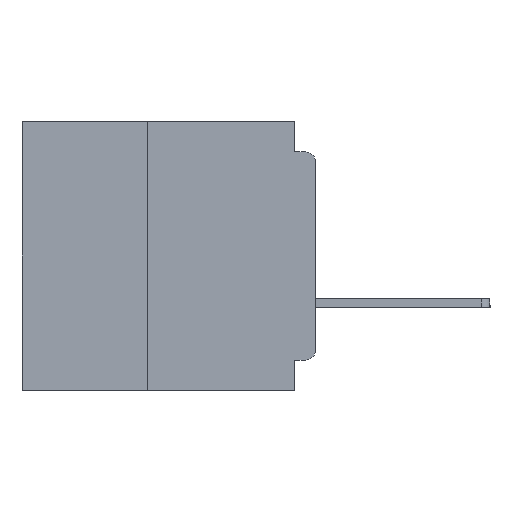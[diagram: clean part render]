
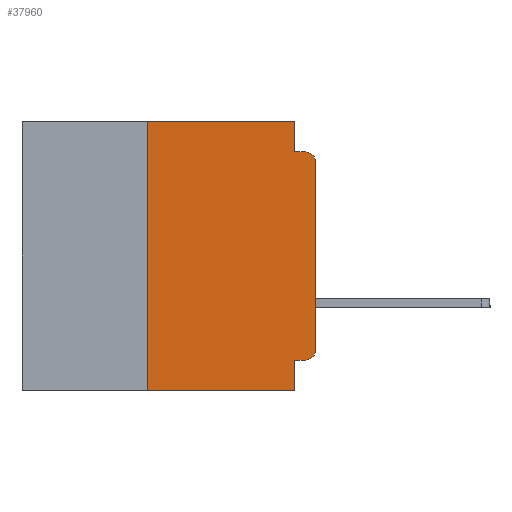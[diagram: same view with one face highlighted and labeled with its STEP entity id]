
A CAD part, left-side view. The second image highlights one B-rep face of the part: STEP entity #37960.
In plain terms, the highlighted planar face has unit normal (-1, 0, 0).
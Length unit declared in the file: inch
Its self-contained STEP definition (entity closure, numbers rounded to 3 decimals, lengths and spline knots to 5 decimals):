
#491 = ORIENTED_EDGE ( 'NONE', *, *, #46022, .F. ) ;
#1719 = VECTOR ( 'NONE', #11478, 39.37008 ) ;
#2384 = DIRECTION ( 'NONE',  ( 0., 1., 0. ) ) ;
#2435 = DIRECTION ( 'NONE',  ( 1., 0., 0. ) ) ;
#2574 = CARTESIAN_POINT ( 'NONE',  ( 0., 0., -0.355 ) ) ;
#2747 = VERTEX_POINT ( 'NONE', #2765 ) ;
#2765 = CARTESIAN_POINT ( 'NONE',  ( 0., 0., -0.34 ) ) ;
#3099 = DIRECTION ( 'NONE',  ( 0., -1., 0. ) ) ;
#3455 = CARTESIAN_POINT ( 'NONE',  ( 0., 0., -0.06 ) ) ;
#4271 = CIRCLE ( 'NONE', #40522, 0.015 ) ;
#4437 = EDGE_CURVE ( 'NONE', #35817, #33585, #36185, .T. ) ;
#5248 = VECTOR ( 'NONE', #12627, 39.37008 ) ;
#5250 = LINE ( 'NONE', #28716, #26916 ) ;
#6099 = VERTEX_POINT ( 'NONE', #3455 ) ;
#6126 = EDGE_CURVE ( 'NONE', #36416, #35817, #7019, .T. ) ;
#6572 = DIRECTION ( 'NONE',  ( 0., 0., 1. ) ) ;
#7019 = LINE ( 'NONE', #2574, #50005 ) ;
#8193 = EDGE_LOOP ( 'NONE', ( #16247, #42101, #491, #33173, #20647, #9060, #18084, #15968, #11695, #17584 ) ) ;
#9060 = ORIENTED_EDGE ( 'NONE', *, *, #16809, .F. ) ;
#10268 = PLANE ( 'NONE',  #50622 ) ;
#10523 = EDGE_CURVE ( 'NONE', #38878, #30469, #30773, .T. ) ;
#11369 = VERTEX_POINT ( 'NONE', #50577 ) ;
#11478 = DIRECTION ( 'NONE',  ( 0., 0., -1. ) ) ;
#11664 = CARTESIAN_POINT ( 'NONE',  ( 0., 0.031, -0.4 ) ) ;
#11695 = ORIENTED_EDGE ( 'NONE', *, *, #6126, .F. ) ;
#12627 = DIRECTION ( 'NONE',  ( 0., 0., 1. ) ) ;
#15305 = EDGE_CURVE ( 'NONE', #2747, #6099, #38279, .T. ) ;
#15968 = ORIENTED_EDGE ( 'NONE', *, *, #4437, .F. ) ;
#16247 = ORIENTED_EDGE ( 'NONE', *, *, #15305, .T. ) ;
#16809 = EDGE_CURVE ( 'NONE', #19910, #42015, #19334, .T. ) ;
#17584 = ORIENTED_EDGE ( 'NONE', *, *, #44099, .T. ) ;
#18084 = ORIENTED_EDGE ( 'NONE', *, *, #33941, .T. ) ;
#18646 = CARTESIAN_POINT ( 'NONE',  ( 0., 0.031, -0.045 ) ) ;
#19334 = LINE ( 'NONE', #24014, #29425 ) ;
#19910 = VERTEX_POINT ( 'NONE', #29352 ) ;
#20647 = ORIENTED_EDGE ( 'NONE', *, *, #38641, .F. ) ;
#20707 = VECTOR ( 'NONE', #3099, 39.37008 ) ;
#21004 = VECTOR ( 'NONE', #37143, 39.37008 ) ;
#23103 = CARTESIAN_POINT ( 'NONE',  ( 0., 0.015, -0.06 ) ) ;
#24014 = CARTESIAN_POINT ( 'NONE',  ( 0., 0.25, -0.4 ) ) ;
#24723 = CARTESIAN_POINT ( 'NONE',  ( 0., 0.437, -0.4 ) ) ;
#24747 = DIRECTION ( 'NONE',  ( -1., 0., 0. ) ) ;
#26424 = CARTESIAN_POINT ( 'NONE',  ( 0., 0.031, -0.4 ) ) ;
#26916 = VECTOR ( 'NONE', #32986, 39.37008 ) ;
#27395 = DIRECTION ( 'NONE',  ( 0., 0., -1. ) ) ;
#27519 = DIRECTION ( 'NONE',  ( 0., 0., -1. ) ) ;
#28716 = CARTESIAN_POINT ( 'NONE',  ( 0., 0.437, 0. ) ) ;
#29352 = CARTESIAN_POINT ( 'NONE',  ( 0., 0.25, -0.4 ) ) ;
#29425 = VECTOR ( 'NONE', #6572, 39.37008 ) ;
#30469 = VERTEX_POINT ( 'NONE', #18646 ) ;
#30773 = LINE ( 'NONE', #36122, #53427 ) ;
#31906 = CIRCLE ( 'NONE', #35535, 0.015 ) ;
#32410 = LINE ( 'NONE', #45559, #21004 ) ;
#32686 = DIRECTION ( 'NONE',  ( 0., 0., -1. ) ) ;
#32821 = CARTESIAN_POINT ( 'NONE',  ( 0., 0.015, -0.355 ) ) ;
#32986 = DIRECTION ( 'NONE',  ( 0., -1., 0. ) ) ;
#33036 = FACE_OUTER_BOUND ( 'NONE', #8193, .T. ) ;
#33173 = ORIENTED_EDGE ( 'NONE', *, *, #10523, .F. ) ;
#33253 = CARTESIAN_POINT ( 'NONE',  ( 0., 0.25, 0. ) ) ;
#33585 = VERTEX_POINT ( 'NONE', #26424 ) ;
#33941 = EDGE_CURVE ( 'NONE', #19910, #33585, #54788, .T. ) ;
#34053 = CARTESIAN_POINT ( 'NONE',  ( 0., 0., 0. ) ) ;
#35535 = AXIS2_PLACEMENT_3D ( 'NONE', #23103, #52923, #27395 ) ;
#35817 = VERTEX_POINT ( 'NONE', #45963 ) ;
#36038 = CARTESIAN_POINT ( 'NONE',  ( 0., 0.437, 0. ) ) ;
#36122 = CARTESIAN_POINT ( 'NONE',  ( 0., 0.031, 0. ) ) ;
#36185 = LINE ( 'NONE', #11664, #1719 ) ;
#36416 = VERTEX_POINT ( 'NONE', #32821 ) ;
#37143 = DIRECTION ( 'NONE',  ( 0., -1., 0. ) ) ;
#37960 = ADVANCED_FACE ( 'NONE', ( #33036 ), #10268, .F. ) ;
#38279 = LINE ( 'NONE', #34053, #5248 ) ;
#38641 = EDGE_CURVE ( 'NONE', #42015, #38878, #5250, .T. ) ;
#38878 = VERTEX_POINT ( 'NONE', #47341 ) ;
#40522 = AXIS2_PLACEMENT_3D ( 'NONE', #50311, #24747, #54583 ) ;
#42015 = VERTEX_POINT ( 'NONE', #33253 ) ;
#42101 = ORIENTED_EDGE ( 'NONE', *, *, #50895, .T. ) ;
#44099 = EDGE_CURVE ( 'NONE', #36416, #2747, #4271, .T. ) ;
#45559 = CARTESIAN_POINT ( 'NONE',  ( 0., 0., -0.045 ) ) ;
#45963 = CARTESIAN_POINT ( 'NONE',  ( 0., 0.031, -0.355 ) ) ;
#46022 = EDGE_CURVE ( 'NONE', #30469, #11369, #32410, .T. ) ;
#47341 = CARTESIAN_POINT ( 'NONE',  ( 0., 0.031, 0. ) ) ;
#50005 = VECTOR ( 'NONE', #2384, 39.37008 ) ;
#50311 = CARTESIAN_POINT ( 'NONE',  ( 0., 0.015, -0.34 ) ) ;
#50577 = CARTESIAN_POINT ( 'NONE',  ( 0., 0.015, -0.045 ) ) ;
#50622 = AXIS2_PLACEMENT_3D ( 'NONE', #36038, #2435, #32686 ) ;
#50895 = EDGE_CURVE ( 'NONE', #6099, #11369, #31906, .T. ) ;
#52923 = DIRECTION ( 'NONE',  ( -1., 0., 0. ) ) ;
#53427 = VECTOR ( 'NONE', #27519, 39.37008 ) ;
#54583 = DIRECTION ( 'NONE',  ( 0., 0., -1. ) ) ;
#54788 = LINE ( 'NONE', #24723, #20707 ) ;
